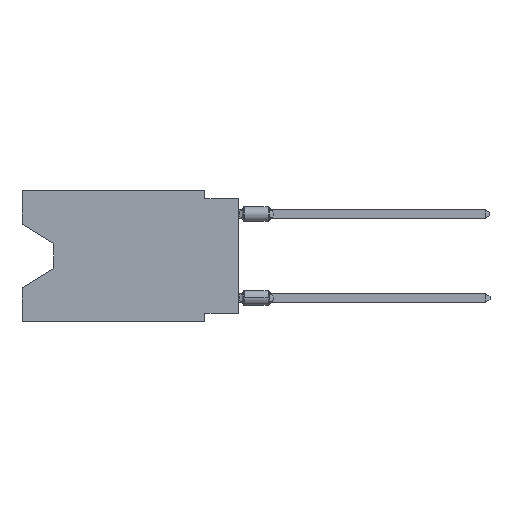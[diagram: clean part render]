
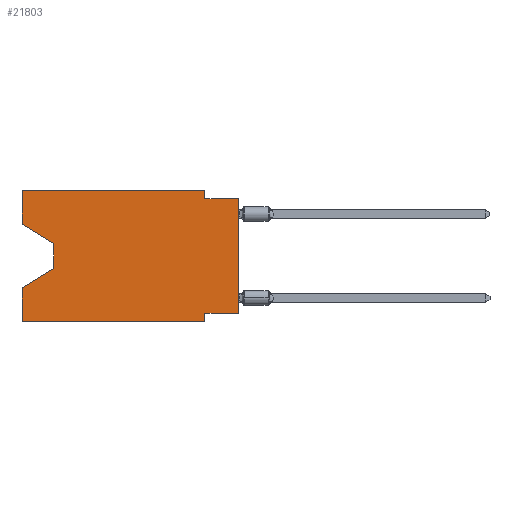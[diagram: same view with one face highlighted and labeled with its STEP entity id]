
A CAD part, left-side view. The second image highlights one B-rep face of the part: STEP entity #21803.
In plain terms, the highlighted planar face has unit normal (-1, 0, 0).
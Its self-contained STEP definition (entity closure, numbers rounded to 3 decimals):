
#25 = CARTESIAN_POINT ( 'NONE',  ( 0., 16.383, 0. ) ) ;
#356 = DIRECTION ( 'NONE',  ( 0., 0., -1. ) ) ;
#467 = EDGE_CURVE ( 'NONE', #22167, #20573, #15801, .T. ) ;
#597 = VERTEX_POINT ( 'NONE', #25741 ) ;
#723 = DIRECTION ( 'NONE',  ( 0., -0.855, -0.519 ) ) ;
#770 = CARTESIAN_POINT ( 'NONE',  ( 0., 0., -0.635 ) ) ;
#844 = CARTESIAN_POINT ( 'NONE',  ( 0., 2.54, -9.906 ) ) ;
#922 = EDGE_CURVE ( 'NONE', #19711, #2462, #25711, .T. ) ;
#1091 = EDGE_CURVE ( 'NONE', #27968, #16953, #9866, .T. ) ;
#1123 = DIRECTION ( 'NONE',  ( 0., -1., 0. ) ) ;
#1361 = CARTESIAN_POINT ( 'NONE',  ( 0., 0., -9.271 ) ) ;
#1811 = LINE ( 'NONE', #1361, #4755 ) ;
#2260 = ORIENTED_EDGE ( 'NONE', *, *, #24028, .F. ) ;
#2462 = VERTEX_POINT ( 'NONE', #11159 ) ;
#2521 = CARTESIAN_POINT ( 'NONE',  ( 0., 16.383, 0. ) ) ;
#2800 = DIRECTION ( 'NONE',  ( 0., 0.855, -0.519 ) ) ;
#3508 = DIRECTION ( 'NONE',  ( 0., -1., 0. ) ) ;
#4536 = EDGE_CURVE ( 'NONE', #597, #27968, #27398, .T. ) ;
#4548 = ORIENTED_EDGE ( 'NONE', *, *, #1091, .F. ) ;
#4739 = LINE ( 'NONE', #5022, #9331 ) ;
#4755 = VECTOR ( 'NONE', #17931, 1000. ) ;
#5022 = CARTESIAN_POINT ( 'NONE',  ( 0., 13.97, -4.013 ) ) ;
#5394 = CARTESIAN_POINT ( 'NONE',  ( 0., 0., -9.271 ) ) ;
#5496 = CARTESIAN_POINT ( 'NONE',  ( 0., 0., -0.635 ) ) ;
#5785 = LINE ( 'NONE', #20211, #12409 ) ;
#6394 = EDGE_CURVE ( 'NONE', #29655, #16953, #27653, .T. ) ;
#6512 = FACE_OUTER_BOUND ( 'NONE', #12361, .T. ) ;
#6638 = ORIENTED_EDGE ( 'NONE', *, *, #7688, .T. ) ;
#6712 = ORIENTED_EDGE ( 'NONE', *, *, #24574, .F. ) ;
#7058 = CARTESIAN_POINT ( 'NONE',  ( 0., 16.383, -2.546 ) ) ;
#7060 = VECTOR ( 'NONE', #2800, 1000. ) ;
#7115 = EDGE_CURVE ( 'NONE', #29655, #22167, #1811, .T. ) ;
#7118 = DIRECTION ( 'NONE',  ( 1., 0., 0. ) ) ;
#7688 = EDGE_CURVE ( 'NONE', #28071, #20573, #23926, .T. ) ;
#7769 = VECTOR ( 'NONE', #723, 1000. ) ;
#8390 = VERTEX_POINT ( 'NONE', #13849 ) ;
#8716 = ORIENTED_EDGE ( 'NONE', *, *, #10143, .T. ) ;
#9208 = ORIENTED_EDGE ( 'NONE', *, *, #20925, .T. ) ;
#9238 = PLANE ( 'NONE',  #23684 ) ;
#9331 = VECTOR ( 'NONE', #356, 1000. ) ;
#9621 = LINE ( 'NONE', #7058, #7769 ) ;
#9866 = LINE ( 'NONE', #5496, #17586 ) ;
#10143 = EDGE_CURVE ( 'NONE', #13048, #8390, #9621, .T. ) ;
#10601 = CARTESIAN_POINT ( 'NONE',  ( 0., 16.383, -2.546 ) ) ;
#10798 = VERTEX_POINT ( 'NONE', #25 ) ;
#11159 = CARTESIAN_POINT ( 'NONE',  ( 0., 16.383, -7.36 ) ) ;
#11594 = ORIENTED_EDGE ( 'NONE', *, *, #4536, .F. ) ;
#11651 = DIRECTION ( 'NONE',  ( 0., 0., 1. ) ) ;
#11992 = DIRECTION ( 'NONE',  ( 0., 0., 1. ) ) ;
#12133 = CARTESIAN_POINT ( 'NONE',  ( 0., 16.383, -9.906 ) ) ;
#12361 = EDGE_LOOP ( 'NONE', ( #8716, #9208, #22636, #2260, #6638, #17051, #21928, #26504, #4548, #11594, #13066, #6712 ) ) ;
#12409 = VECTOR ( 'NONE', #20062, 1000. ) ;
#12820 = CARTESIAN_POINT ( 'NONE',  ( 0., 16.383, 0. ) ) ;
#13048 = VERTEX_POINT ( 'NONE', #10601 ) ;
#13066 = ORIENTED_EDGE ( 'NONE', *, *, #15423, .F. ) ;
#13494 = VECTOR ( 'NONE', #3508, 1000. ) ;
#13849 = CARTESIAN_POINT ( 'NONE',  ( 0., 13.97, -4.013 ) ) ;
#14328 = VECTOR ( 'NONE', #11651, 1000. ) ;
#14557 = LINE ( 'NONE', #2521, #17212 ) ;
#14637 = LINE ( 'NONE', #12820, #13494 ) ;
#15340 = DIRECTION ( 'NONE',  ( 0., 0., -1. ) ) ;
#15423 = EDGE_CURVE ( 'NONE', #10798, #597, #14637, .T. ) ;
#15801 = LINE ( 'NONE', #17616, #26754 ) ;
#16002 = DIRECTION ( 'NONE',  ( 0., 0., -1. ) ) ;
#16953 = VERTEX_POINT ( 'NONE', #770 ) ;
#17051 = ORIENTED_EDGE ( 'NONE', *, *, #467, .F. ) ;
#17212 = VECTOR ( 'NONE', #11992, 1000. ) ;
#17586 = VECTOR ( 'NONE', #1123, 1000. ) ;
#17616 = CARTESIAN_POINT ( 'NONE',  ( 0., 2.54, -9.906 ) ) ;
#17931 = DIRECTION ( 'NONE',  ( 0., 1., 0. ) ) ;
#18483 = CARTESIAN_POINT ( 'NONE',  ( 0., 13.97, -5.893 ) ) ;
#19711 = VERTEX_POINT ( 'NONE', #21398 ) ;
#20062 = DIRECTION ( 'NONE',  ( 0., 0., 1. ) ) ;
#20211 = CARTESIAN_POINT ( 'NONE',  ( 0., 16.383, 0. ) ) ;
#20573 = VERTEX_POINT ( 'NONE', #844 ) ;
#20925 = EDGE_CURVE ( 'NONE', #8390, #19711, #4739, .T. ) ;
#21199 = DIRECTION ( 'NONE',  ( 0., -1., 0. ) ) ;
#21398 = CARTESIAN_POINT ( 'NONE',  ( 0., 13.97, -5.893 ) ) ;
#21803 = ADVANCED_FACE ( 'NONE', ( #6512 ), #9238, .F. ) ;
#21928 = ORIENTED_EDGE ( 'NONE', *, *, #7115, .F. ) ;
#22092 = VECTOR ( 'NONE', #21199, 1000. ) ;
#22167 = VERTEX_POINT ( 'NONE', #24726 ) ;
#22445 = CARTESIAN_POINT ( 'NONE',  ( 0., 2.54, -0.635 ) ) ;
#22636 = ORIENTED_EDGE ( 'NONE', *, *, #922, .T. ) ;
#22714 = CARTESIAN_POINT ( 'NONE',  ( 0., 2.54, 0. ) ) ;
#23126 = CARTESIAN_POINT ( 'NONE',  ( 0., 0., 0. ) ) ;
#23413 = VECTOR ( 'NONE', #27241, 1000. ) ;
#23684 = AXIS2_PLACEMENT_3D ( 'NONE', #25057, #7118, #16002 ) ;
#23926 = LINE ( 'NONE', #12133, #22092 ) ;
#24028 = EDGE_CURVE ( 'NONE', #28071, #2462, #14557, .T. ) ;
#24574 = EDGE_CURVE ( 'NONE', #13048, #10798, #5785, .T. ) ;
#24726 = CARTESIAN_POINT ( 'NONE',  ( 0., 2.54, -9.271 ) ) ;
#25057 = CARTESIAN_POINT ( 'NONE',  ( 0., 16.383, 0. ) ) ;
#25711 = LINE ( 'NONE', #18483, #7060 ) ;
#25741 = CARTESIAN_POINT ( 'NONE',  ( 0., 2.54, 0. ) ) ;
#25899 = CARTESIAN_POINT ( 'NONE',  ( 0., 16.383, -9.906 ) ) ;
#26504 = ORIENTED_EDGE ( 'NONE', *, *, #6394, .T. ) ;
#26754 = VECTOR ( 'NONE', #15340, 1000. ) ;
#27241 = DIRECTION ( 'NONE',  ( 0., 0., -1. ) ) ;
#27398 = LINE ( 'NONE', #22714, #23413 ) ;
#27653 = LINE ( 'NONE', #23126, #14328 ) ;
#27968 = VERTEX_POINT ( 'NONE', #22445 ) ;
#28071 = VERTEX_POINT ( 'NONE', #25899 ) ;
#29655 = VERTEX_POINT ( 'NONE', #5394 ) ;
